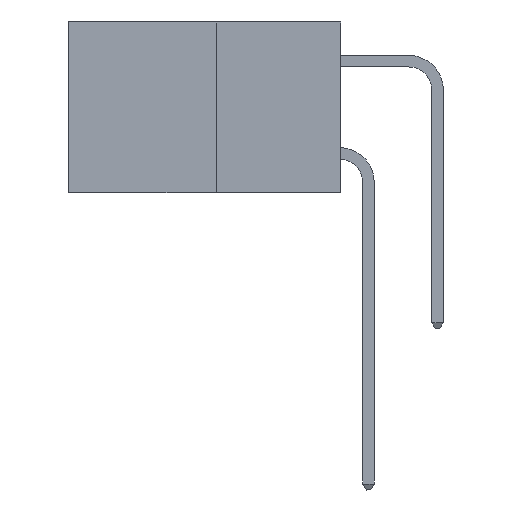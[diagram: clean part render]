
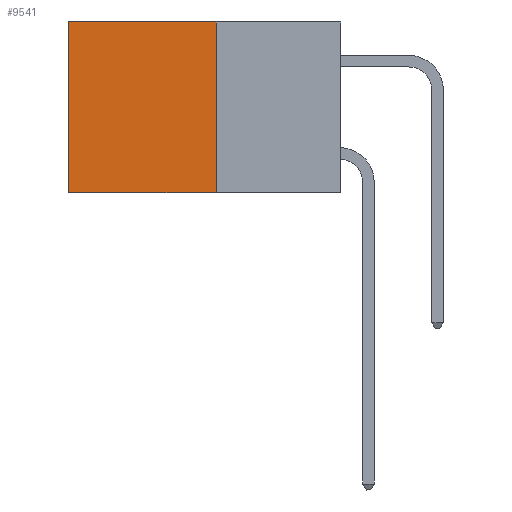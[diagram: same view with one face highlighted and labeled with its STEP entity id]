
A CAD part, left-side view. The second image highlights one B-rep face of the part: STEP entity #9541.
In plain terms, the highlighted planar face has unit normal (-1, 0, 0).
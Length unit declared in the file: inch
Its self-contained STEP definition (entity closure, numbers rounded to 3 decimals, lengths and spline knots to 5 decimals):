
#1003 = LINE ( 'NONE', #6730, #7388 ) ;
#1032 = CARTESIAN_POINT ( 'NONE',  ( 0.277, 0.27, 0. ) ) ;
#2430 = VERTEX_POINT ( 'NONE', #1032 ) ;
#3652 = VECTOR ( 'NONE', #8436, 39.37008 ) ;
#4068 = LINE ( 'NONE', #14699, #3652 ) ;
#5272 = DIRECTION ( 'NONE',  ( 1., 0., 0. ) ) ;
#5792 = EDGE_CURVE ( 'NONE', #12897, #11484, #12405, .T. ) ;
#5825 = LINE ( 'NONE', #7841, #9192 ) ;
#6350 = CARTESIAN_POINT ( 'NONE',  ( 0.277, 0.59, 0. ) ) ;
#6730 = CARTESIAN_POINT ( 'NONE',  ( 0.277, 0.27, -0.37 ) ) ;
#7373 = ORIENTED_EDGE ( 'NONE', *, *, #10515, .T. ) ;
#7388 = VECTOR ( 'NONE', #7977, 39.37008 ) ;
#7841 = CARTESIAN_POINT ( 'NONE',  ( 0.277, 0.59, -0.37 ) ) ;
#7977 = DIRECTION ( 'NONE',  ( 0., 0., -1. ) ) ;
#8436 = DIRECTION ( 'NONE',  ( 0., 1., 0. ) ) ;
#8497 = EDGE_CURVE ( 'NONE', #2430, #12897, #1003, .T. ) ;
#8940 = EDGE_LOOP ( 'NONE', ( #10189, #15051, #9633, #7373 ) ) ;
#9192 = VECTOR ( 'NONE', #11607, 39.37008 ) ;
#9483 = VECTOR ( 'NONE', #16050, 39.37008 ) ;
#9541 = ADVANCED_FACE ( 'NONE', ( #11297 ), #10253, .F. ) ;
#9633 = ORIENTED_EDGE ( 'NONE', *, *, #8497, .F. ) ;
#10189 = ORIENTED_EDGE ( 'NONE', *, *, #14684, .T. ) ;
#10253 = PLANE ( 'NONE',  #10926 ) ;
#10515 = EDGE_CURVE ( 'NONE', #2430, #13757, #4068, .T. ) ;
#10926 = AXIS2_PLACEMENT_3D ( 'NONE', #12761, #5272, #14004 ) ;
#11297 = FACE_OUTER_BOUND ( 'NONE', #8940, .T. ) ;
#11484 = VERTEX_POINT ( 'NONE', #14941 ) ;
#11607 = DIRECTION ( 'NONE',  ( 0., 0., -1. ) ) ;
#12405 = LINE ( 'NONE', #12653, #9483 ) ;
#12653 = CARTESIAN_POINT ( 'NONE',  ( 0.277, 0.27, -0.37 ) ) ;
#12761 = CARTESIAN_POINT ( 'NONE',  ( 0.277, 0.27, -0.37 ) ) ;
#12897 = VERTEX_POINT ( 'NONE', #13706 ) ;
#13706 = CARTESIAN_POINT ( 'NONE',  ( 0.277, 0.27, -0.37 ) ) ;
#13757 = VERTEX_POINT ( 'NONE', #6350 ) ;
#14004 = DIRECTION ( 'NONE',  ( 0., 0., -1. ) ) ;
#14684 = EDGE_CURVE ( 'NONE', #13757, #11484, #5825, .T. ) ;
#14699 = CARTESIAN_POINT ( 'NONE',  ( 0.277, 0.27, 0. ) ) ;
#14941 = CARTESIAN_POINT ( 'NONE',  ( 0.277, 0.59, -0.37 ) ) ;
#15051 = ORIENTED_EDGE ( 'NONE', *, *, #5792, .F. ) ;
#16050 = DIRECTION ( 'NONE',  ( 0., 1., 0. ) ) ;
